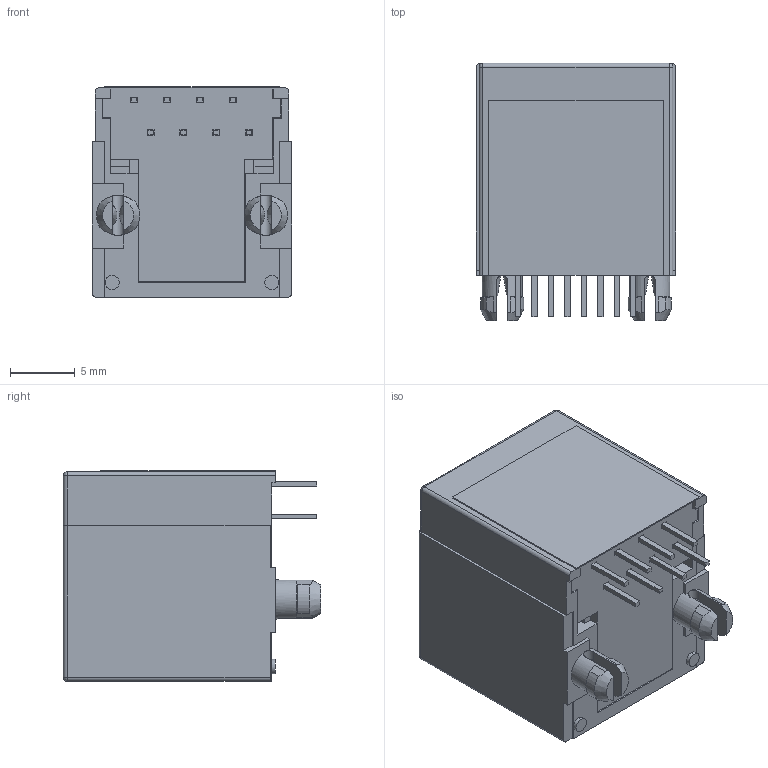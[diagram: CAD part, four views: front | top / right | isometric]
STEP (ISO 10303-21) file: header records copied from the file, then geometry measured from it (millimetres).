
FILE_DESCRIPTION (( 'STEP AP203' ), '1' );
FILE_NAME ('RJ2K018821P00931.STEP', '2019-12-13T19:31:08', ( '' ), ( '' ), 'SwSTEP 2.0', 'SolidWorks 2016', '' );
FILE_SCHEMA (( 'CONFIG_CONTROL_DESIGN' ));
Length unit declared in the file: millimetre
Products named in the file (5): RJ2K018821P00931; 2K Mylar Tape; 2K Contact Lock; 2K Insulator; 2K Contacts
Assembly tree (4 placements, depth 2):
  RJ2K018821P00931
    2K Insulator
    2K Contacts
    2K Contact Lock
    2K Mylar Tape
Bounding box: 15.4 x 19.9 x 16.3 mm (x, y, z)
Volume: 2490.9 mm3; surface area: 4331.5 mm2
Topology: 11 solids, 11 shells, 729 faces, 2072 edges, 1347 vertices
Faces by surface type: plane 592, cylinder 113, bspline 12, cone 8, sphere 4
Entity records: 24120 total; most frequent: CARTESIAN_POINT 4828, ORIENTED_EDGE 4128, DIRECTION 3593, EDGE_CURVE 2064, VECTOR 1773, LINE 1773, VERTEX_POINT 1347, AXIS2_PLACEMENT_3D 910
